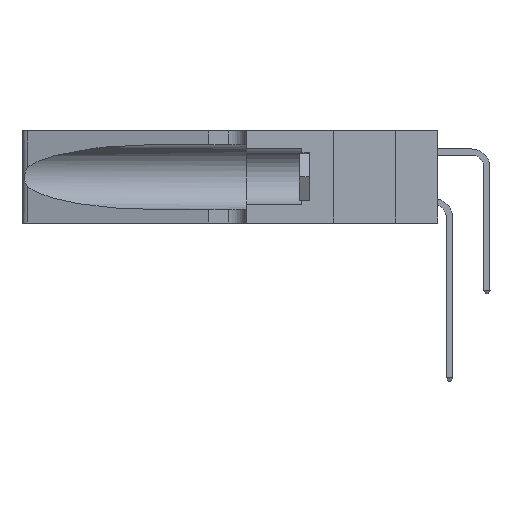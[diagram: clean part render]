
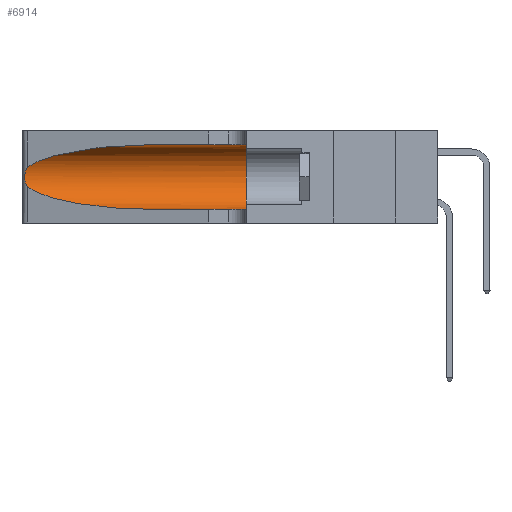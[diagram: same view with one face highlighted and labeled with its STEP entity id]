
A CAD part, left-side view. The second image highlights one B-rep face of the part: STEP entity #6914.
In plain terms, the highlighted cylindrical face has radius 3.308 mm (diameter 6.617 mm), a partial arc.
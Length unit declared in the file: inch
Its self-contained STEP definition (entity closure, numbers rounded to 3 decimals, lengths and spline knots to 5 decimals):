
#468 = CARTESIAN_POINT ( 'NONE',  ( 0.1305, 1.61858, 0.05475 ) ) ;
#1194 = CARTESIAN_POINT ( 'NONE',  ( 0.1305, 1.61858, 0.185 ) ) ;
#1746 = VECTOR ( 'NONE', #3961, 39.37008 ) ;
#3202 = CARTESIAN_POINT ( 'NONE',  ( 0.1305, 0.72297, 0.31525 ) ) ;
#3348 = CARTESIAN_POINT ( 'NONE',  ( 0.25487, 1.22718, 0.22369 ) ) ;
#3441 = CARTESIAN_POINT ( 'NONE',  ( 0.1305, 0.72297, 0.05475 ) ) ;
#3961 = DIRECTION ( 'NONE',  ( 0., -1., 0. ) ) ;
#4691 = DIRECTION ( 'NONE',  ( 0., 0., -1. ) ) ;
#4969 = CARTESIAN_POINT ( 'NONE',  ( 0.25487, 1.22718, 0.14631 ) ) ;
#5878 = CARTESIAN_POINT ( 'NONE',  ( 0.25854, 1.2359, 0.20912 ) ) ;
#6857 = ORIENTED_EDGE ( 'NONE', *, *, #34839, .T. ) ;
#6914 = ADVANCED_FACE ( 'NONE', ( #23054 ), #21982, .F. ) ;
#7942 = EDGE_CURVE ( 'NONE', #24556, #14615, #27279, .T. ) ;
#8475 = CARTESIAN_POINT ( 'NONE',  ( 0.1305, 0.35, 0.31525 ) ) ;
#9364 = CARTESIAN_POINT ( 'NONE',  ( 0.26075, 1.23896, 0.19203 ) ) ;
#9746 = CARTESIAN_POINT ( 'NONE',  ( 0.2373, 1.15595, 0.08982 ) ) ;
#9880 = EDGE_CURVE ( 'NONE', #21106, #24556, #43498, .T. ) ;
#10456 = EDGE_CURVE ( 'NONE', #37037, #11998, #37081, .T. ) ;
#11052 = AXIS2_PLACEMENT_3D ( 'NONE', #40415, #20211, #43777 ) ;
#11998 = VERTEX_POINT ( 'NONE', #4969 ) ;
#12833 = CARTESIAN_POINT ( 'NONE',  ( 0.26017, 1.23833, 0.17102 ) ) ;
#13208 = CARTESIAN_POINT ( 'NONE',  ( 0.1305, 0.72297, 0.05475 ) ) ;
#14615 = VERTEX_POINT ( 'NONE', #19060 ) ;
#14880 =( BOUNDED_CURVE ( )  B_SPLINE_CURVE ( 3, ( #3202, #40511, #23854, #3348 ),
 .UNSPECIFIED., .F., .T. ) 
 B_SPLINE_CURVE_WITH_KNOTS ( ( 4, 4 ),
 ( 1.5708, 2.84003 ),
 .UNSPECIFIED. ) 
 CURVE ( )  GEOMETRIC_REPRESENTATION_ITEM ( )  RATIONAL_B_SPLINE_CURVE ( ( 1., 0.87, 0.87, 1. ) ) 
 REPRESENTATION_ITEM ( '' )  );
#16271 = CARTESIAN_POINT ( 'NONE',  ( 0.25789, 1.23486, 0.15765 ) ) ;
#19060 = CARTESIAN_POINT ( 'NONE',  ( 0.1305, 0.35, 0.05475 ) ) ;
#19673 = CARTESIAN_POINT ( 'NONE',  ( 0.25555, 1.22993, 0.14849 ) ) ;
#19747 = CARTESIAN_POINT ( 'NONE',  ( 0.1305, 0.72297, 0.31525 ) ) ;
#20211 = DIRECTION ( 'NONE',  ( 0., 1., 0. ) ) ;
#21106 = VERTEX_POINT ( 'NONE', #19747 ) ;
#21982 = CYLINDRICAL_SURFACE ( 'NONE', #37123, 0.13025 ) ;
#22260 = ORIENTED_EDGE ( 'NONE', *, *, #9880, .F. ) ;
#22944 = CARTESIAN_POINT ( 'NONE',  ( 0.25487, 1.22718, 0.22369 ) ) ;
#23046 = ORIENTED_EDGE ( 'NONE', *, *, #39245, .T. ) ;
#23054 = FACE_OUTER_BOUND ( 'NONE', #27784, .T. ) ;
#23576 = CARTESIAN_POINT ( 'NONE',  ( 0.1305, 1.61858, 0.31525 ) ) ;
#23854 = CARTESIAN_POINT ( 'NONE',  ( 0.2373, 1.15595, 0.28018 ) ) ;
#24548 = VECTOR ( 'NONE', #43733, 39.37008 ) ;
#24556 = VERTEX_POINT ( 'NONE', #8475 ) ;
#25165 = DIRECTION ( 'NONE',  ( 0., -1., 0. ) ) ;
#26005 = ORIENTED_EDGE ( 'NONE', *, *, #7942, .F. ) ;
#26328 = CARTESIAN_POINT ( 'NONE',  ( 0.25787, 1.23484, 0.2124 ) ) ;
#27279 = CIRCLE ( 'NONE', #11052, 0.13025 ) ;
#27784 = EDGE_LOOP ( 'NONE', ( #23046, #32399, #34845, #6857, #26005, #22260 ) ) ;
#28998 = LINE ( 'NONE', #468, #1746 ) ;
#29401 = CARTESIAN_POINT ( 'NONE',  ( 0.25639, 1.23184, 0.21858 ) ) ;
#29691 = CARTESIAN_POINT ( 'NONE',  ( 0.26018, 1.23835, 0.19895 ) ) ;
#30063 = CARTESIAN_POINT ( 'NONE',  ( 0.25487, 1.22718, 0.14631 ) ) ;
#32399 = ORIENTED_EDGE ( 'NONE', *, *, #10456, .T. ) ;
#33075 = CARTESIAN_POINT ( 'NONE',  ( 0.26075, 1.23896, 0.178 ) ) ;
#33448 = CARTESIAN_POINT ( 'NONE',  ( 0.18966, 0.96281, 0.05475 ) ) ;
#34839 = EDGE_CURVE ( 'NONE', #37720, #14615, #28998, .T. ) ;
#34845 = ORIENTED_EDGE ( 'NONE', *, *, #36383, .T. ) ;
#36383 = EDGE_CURVE ( 'NONE', #11998, #37720, #38443, .T. ) ;
#36466 = CARTESIAN_POINT ( 'NONE',  ( 0.25856, 1.23593, 0.16098 ) ) ;
#37037 = VERTEX_POINT ( 'NONE', #43728 ) ;
#37081 = B_SPLINE_CURVE_WITH_KNOTS ( 'NONE', 3,
 ( #22944, #39580, #29401, #26328, #5878, #29691, #9364, #33075, #12833, #36466, #16271, #39875, #19673, #43249 ),
 .UNSPECIFIED., .F., .F.,
 ( 4, 2, 2, 2, 2, 2, 4 ),
 ( 0., 0.00027, 0.00053, 0.00107, 0.0016, 0.00187, 0.00214 ),
 .UNSPECIFIED. ) ;
#37123 = AXIS2_PLACEMENT_3D ( 'NONE', #1194, #25165, #4691 ) ;
#37720 = VERTEX_POINT ( 'NONE', #3441 ) ;
#38443 =( BOUNDED_CURVE ( )  B_SPLINE_CURVE ( 3, ( #30063, #9746, #33448, #13208 ),
 .UNSPECIFIED., .F., .T. ) 
 B_SPLINE_CURVE_WITH_KNOTS ( ( 4, 4 ),
 ( 3.44316, 4.71239 ),
 .UNSPECIFIED. ) 
 CURVE ( )  GEOMETRIC_REPRESENTATION_ITEM ( )  RATIONAL_B_SPLINE_CURVE ( ( 1., 0.87, 0.87, 1. ) ) 
 REPRESENTATION_ITEM ( '' )  );
#39245 = EDGE_CURVE ( 'NONE', #21106, #37037, #14880, .T. ) ;
#39580 = CARTESIAN_POINT ( 'NONE',  ( 0.25555, 1.22994, 0.2215 ) ) ;
#39875 = CARTESIAN_POINT ( 'NONE',  ( 0.25639, 1.23186, 0.15144 ) ) ;
#40415 = CARTESIAN_POINT ( 'NONE',  ( 0.1305, 0.35, 0.185 ) ) ;
#40511 = CARTESIAN_POINT ( 'NONE',  ( 0.18966, 0.96281, 0.31525 ) ) ;
#43249 = CARTESIAN_POINT ( 'NONE',  ( 0.25487, 1.22718, 0.14631 ) ) ;
#43498 = LINE ( 'NONE', #23576, #24548 ) ;
#43728 = CARTESIAN_POINT ( 'NONE',  ( 0.25487, 1.22718, 0.22369 ) ) ;
#43733 = DIRECTION ( 'NONE',  ( 0., -1., 0. ) ) ;
#43777 = DIRECTION ( 'NONE',  ( 0., 0., 1. ) ) ;
